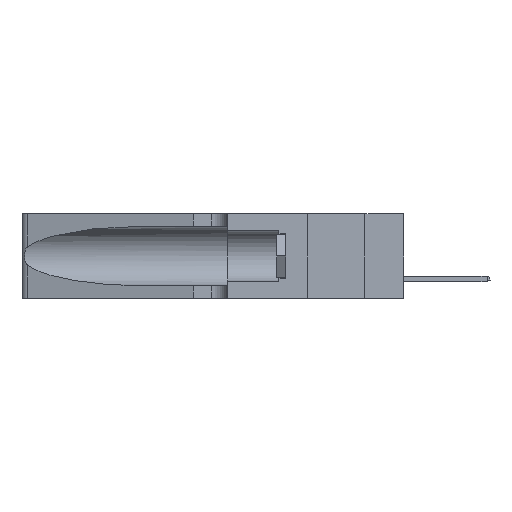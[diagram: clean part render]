
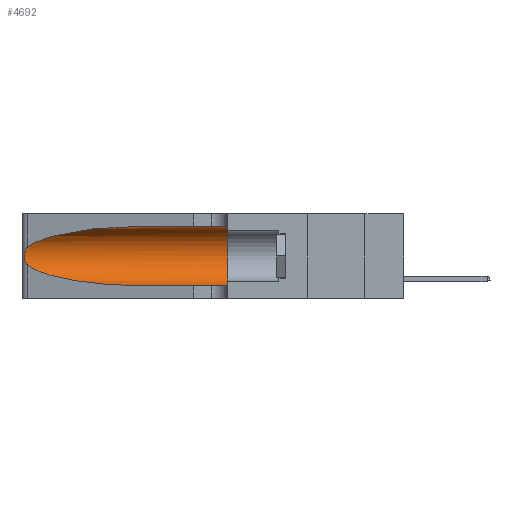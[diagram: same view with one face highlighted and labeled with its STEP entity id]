
A CAD part, left-side view. The second image highlights one B-rep face of the part: STEP entity #4692.
In plain terms, the highlighted cylindrical face has radius 3.308 mm (diameter 6.617 mm), a partial arc.
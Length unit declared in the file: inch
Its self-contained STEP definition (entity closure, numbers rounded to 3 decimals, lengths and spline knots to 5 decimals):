
#222 = EDGE_LOOP ( 'NONE', ( #29707, #36190, #19051, #19055, #36716, #7630 ) ) ;
#686 = CARTESIAN_POINT ( 'NONE',  ( 0.1305, 1.61858, 0.05475 ) ) ;
#1112 =( BOUNDED_CURVE ( )  B_SPLINE_CURVE ( 3, ( #3859, #7077, #19213, #7228 ),
 .UNSPECIFIED., .F., .T. ) 
 B_SPLINE_CURVE_WITH_KNOTS ( ( 4, 4 ),
 ( 3.44316, 4.71239 ),
 .UNSPECIFIED. ) 
 CURVE ( )  GEOMETRIC_REPRESENTATION_ITEM ( )  RATIONAL_B_SPLINE_CURVE ( ( 1., 0.87, 0.87, 1. ) ) 
 REPRESENTATION_ITEM ( '' )  );
#1887 =( BOUNDED_CURVE ( )  B_SPLINE_CURVE ( 3, ( #34894, #23212, #32209, #19747 ),
 .UNSPECIFIED., .F., .F. ) 
 B_SPLINE_CURVE_WITH_KNOTS ( ( 4, 4 ),
 ( 1.5708, 2.84003 ),
 .UNSPECIFIED. ) 
 CURVE ( )  GEOMETRIC_REPRESENTATION_ITEM ( )  RATIONAL_B_SPLINE_CURVE ( ( 1., 0.87, 0.87, 1. ) ) 
 REPRESENTATION_ITEM ( '' )  );
#3610 = CARTESIAN_POINT ( 'NONE',  ( 0.25555, 1.22994, 0.2215 ) ) ;
#3859 = CARTESIAN_POINT ( 'NONE',  ( 0.25487, 1.22718, 0.14631 ) ) ;
#4028 = CARTESIAN_POINT ( 'NONE',  ( 0.25487, 1.22718, 0.22369 ) ) ;
#4675 = EDGE_CURVE ( 'NONE', #9369, #13663, #25032, .T. ) ;
#4692 = ADVANCED_FACE ( 'NONE', ( #32693 ), #35092, .F. ) ;
#6335 = DIRECTION ( 'NONE',  ( 0., 1., 0. ) ) ;
#7077 = CARTESIAN_POINT ( 'NONE',  ( 0.2373, 1.15595, 0.08982 ) ) ;
#7228 = CARTESIAN_POINT ( 'NONE',  ( 0.1305, 0.72297, 0.05475 ) ) ;
#7630 = ORIENTED_EDGE ( 'NONE', *, *, #22514, .F. ) ;
#9369 = VERTEX_POINT ( 'NONE', #10657 ) ;
#9663 = CARTESIAN_POINT ( 'NONE',  ( 0.26017, 1.23833, 0.17102 ) ) ;
#10657 = CARTESIAN_POINT ( 'NONE',  ( 0.1305, 0.35, 0.31525 ) ) ;
#11324 = EDGE_CURVE ( 'NONE', #26624, #15601, #30201, .T. ) ;
#11882 = CARTESIAN_POINT ( 'NONE',  ( 0.25487, 1.22718, 0.14631 ) ) ;
#12583 = CARTESIAN_POINT ( 'NONE',  ( 0.25555, 1.22993, 0.14849 ) ) ;
#12606 = DIRECTION ( 'NONE',  ( 0., -1., 0. ) ) ;
#13094 = CARTESIAN_POINT ( 'NONE',  ( 0.1305, 1.61858, 0.31525 ) ) ;
#13663 = VERTEX_POINT ( 'NONE', #17197 ) ;
#15409 = EDGE_CURVE ( 'NONE', #26391, #26624, #1887, .T. ) ;
#15601 = VERTEX_POINT ( 'NONE', #11882 ) ;
#15648 = CARTESIAN_POINT ( 'NONE',  ( 0.25787, 1.23484, 0.2124 ) ) ;
#15677 = CARTESIAN_POINT ( 'NONE',  ( 0.1305, 0.35, 0.185 ) ) ;
#15789 = DIRECTION ( 'NONE',  ( 0., 0., -1. ) ) ;
#16042 = CARTESIAN_POINT ( 'NONE',  ( 0.25487, 1.22718, 0.14631 ) ) ;
#17197 = CARTESIAN_POINT ( 'NONE',  ( 0.1305, 0.35, 0.05475 ) ) ;
#18225 = AXIS2_PLACEMENT_3D ( 'NONE', #18372, #12606, #15789 ) ;
#18372 = CARTESIAN_POINT ( 'NONE',  ( 0.1305, 1.61858, 0.185 ) ) ;
#18714 = CARTESIAN_POINT ( 'NONE',  ( 0.26075, 1.23896, 0.178 ) ) ;
#19051 = ORIENTED_EDGE ( 'NONE', *, *, #25244, .T. ) ;
#19055 = ORIENTED_EDGE ( 'NONE', *, *, #21990, .T. ) ;
#19213 = CARTESIAN_POINT ( 'NONE',  ( 0.18966, 0.96281, 0.05475 ) ) ;
#19531 = LINE ( 'NONE', #13094, #28020 ) ;
#19747 = CARTESIAN_POINT ( 'NONE',  ( 0.25487, 1.22718, 0.22369 ) ) ;
#21479 = LINE ( 'NONE', #686, #22432 ) ;
#21783 = CARTESIAN_POINT ( 'NONE',  ( 0.25639, 1.23184, 0.21858 ) ) ;
#21990 = EDGE_CURVE ( 'NONE', #30819, #13663, #21479, .T. ) ;
#22332 = CARTESIAN_POINT ( 'NONE',  ( 0.26075, 1.23896, 0.19203 ) ) ;
#22432 = VECTOR ( 'NONE', #25114, 39.37008 ) ;
#22514 = EDGE_CURVE ( 'NONE', #26391, #9369, #19531, .T. ) ;
#22992 = CARTESIAN_POINT ( 'NONE',  ( 0.1305, 0.72297, 0.31525 ) ) ;
#23212 = CARTESIAN_POINT ( 'NONE',  ( 0.18966, 0.96281, 0.31525 ) ) ;
#24836 = CARTESIAN_POINT ( 'NONE',  ( 0.25789, 1.23486, 0.15765 ) ) ;
#25032 = CIRCLE ( 'NONE', #31940, 0.13025 ) ;
#25088 = CARTESIAN_POINT ( 'NONE',  ( 0.25639, 1.23186, 0.15144 ) ) ;
#25114 = DIRECTION ( 'NONE',  ( 0., -1., 0. ) ) ;
#25190 = DIRECTION ( 'NONE',  ( 0., -1., 0. ) ) ;
#25244 = EDGE_CURVE ( 'NONE', #15601, #30819, #1112, .T. ) ;
#26391 = VERTEX_POINT ( 'NONE', #22992 ) ;
#26616 = CARTESIAN_POINT ( 'NONE',  ( 0.1305, 0.72297, 0.05475 ) ) ;
#26624 = VERTEX_POINT ( 'NONE', #36104 ) ;
#28020 = VECTOR ( 'NONE', #25190, 39.37008 ) ;
#29707 = ORIENTED_EDGE ( 'NONE', *, *, #15409, .T. ) ;
#30201 = B_SPLINE_CURVE_WITH_KNOTS ( 'NONE', 3,
 ( #4028, #3610, #21783, #15648, #34268, #33995, #22332, #18714, #9663, #31033, #24836, #25088, #12583, #16042 ),
 .UNSPECIFIED., .F., .F.,
 ( 4, 2, 2, 2, 2, 2, 4 ),
 ( 0., 0.00027, 0.00053, 0.00107, 0.0016, 0.00187, 0.00214 ),
 .UNSPECIFIED. ) ;
#30819 = VERTEX_POINT ( 'NONE', #26616 ) ;
#31033 = CARTESIAN_POINT ( 'NONE',  ( 0.25856, 1.23593, 0.16098 ) ) ;
#31940 = AXIS2_PLACEMENT_3D ( 'NONE', #15677, #6335, #36966 ) ;
#32209 = CARTESIAN_POINT ( 'NONE',  ( 0.2373, 1.15595, 0.28018 ) ) ;
#32693 = FACE_OUTER_BOUND ( 'NONE', #222, .T. ) ;
#33995 = CARTESIAN_POINT ( 'NONE',  ( 0.26018, 1.23835, 0.19895 ) ) ;
#34268 = CARTESIAN_POINT ( 'NONE',  ( 0.25854, 1.2359, 0.20912 ) ) ;
#34894 = CARTESIAN_POINT ( 'NONE',  ( 0.1305, 0.72297, 0.31525 ) ) ;
#35092 = CYLINDRICAL_SURFACE ( 'NONE', #18225, 0.13025 ) ;
#36104 = CARTESIAN_POINT ( 'NONE',  ( 0.25487, 1.22718, 0.22369 ) ) ;
#36190 = ORIENTED_EDGE ( 'NONE', *, *, #11324, .T. ) ;
#36716 = ORIENTED_EDGE ( 'NONE', *, *, #4675, .F. ) ;
#36966 = DIRECTION ( 'NONE',  ( 0., 0., 1. ) ) ;
